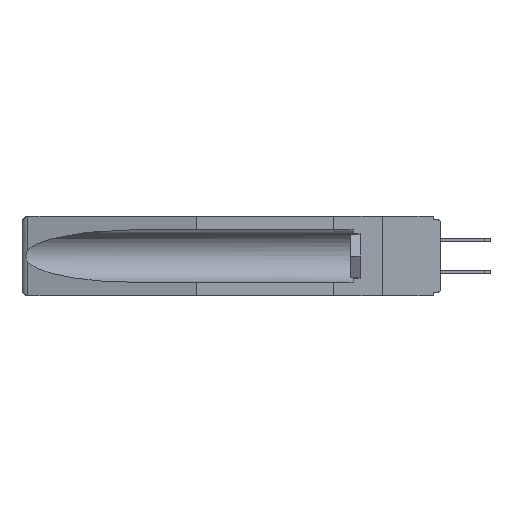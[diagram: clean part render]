
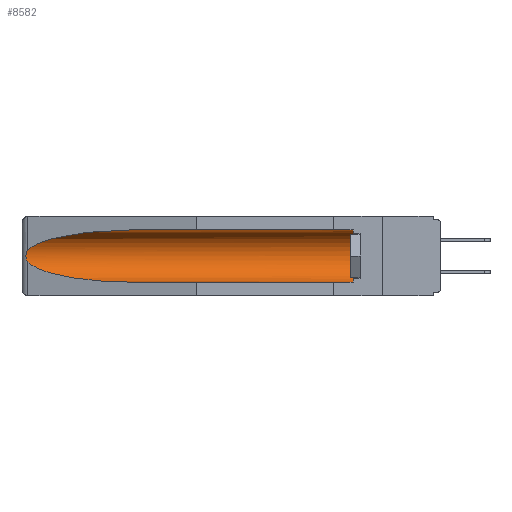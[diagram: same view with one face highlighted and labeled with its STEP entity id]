
A CAD part, left-side view. The second image highlights one B-rep face of the part: STEP entity #8582.
In plain terms, the highlighted cylindrical face has radius 2.857 mm (diameter 5.715 mm), a partial arc.
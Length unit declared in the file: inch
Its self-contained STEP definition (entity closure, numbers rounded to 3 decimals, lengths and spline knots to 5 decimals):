
#1627 = DIRECTION ( 'NONE',  ( 0., -1., 0. ) ) ;
#1773 = CARTESIAN_POINT ( 'NONE',  ( 0.155, -0.30754, -0.1715 ) ) ;
#2093 = AXIS2_PLACEMENT_3D ( 'NONE', #16883, #1627, #15535 ) ;
#2105 = LINE ( 'NONE', #9379, #15382 ) ;
#2114 = CARTESIAN_POINT ( 'NONE',  ( 0.21114, 1.30732, -0.059 ) ) ;
#2133 = CARTESIAN_POINT ( 'NONE',  ( 0.26597, 1.52961, -0.15275 ) ) ;
#2170 = FACE_OUTER_BOUND ( 'NONE', #7596, .T. ) ;
#2476 =( BOUNDED_CURVE ( )  B_SPLINE_CURVE ( 3, ( #14706, #4931, #17585, #3435 ),
 .UNSPECIFIED., .F., .F. ) 
 B_SPLINE_CURVE_WITH_KNOTS ( ( 4, 4 ),
 ( 0.1948, 1.5708 ),
 .UNSPECIFIED. ) 
 CURVE ( )  GEOMETRIC_REPRESENTATION_ITEM ( )  RATIONAL_B_SPLINE_CURVE ( ( 1., 0.848, 0.848, 1. ) ) 
 REPRESENTATION_ITEM ( '' )  );
#2483 = EDGE_CURVE ( 'NONE', #9622, #3540, #13311, .T. ) ;
#2827 = ORIENTED_EDGE ( 'NONE', *, *, #14775, .T. ) ;
#2830 = CYLINDRICAL_SURFACE ( 'NONE', #15640, 0.1125 ) ;
#3435 = CARTESIAN_POINT ( 'NONE',  ( 0.155, 1.07973, -0.284 ) ) ;
#3485 = CARTESIAN_POINT ( 'NONE',  ( 0.26537, 1.52718, -0.19328 ) ) ;
#3540 = VERTEX_POINT ( 'NONE', #5887 ) ;
#3543 = CARTESIAN_POINT ( 'NONE',  ( 0.26654, 1.53092, -0.15636 ) ) ;
#3676 = ORIENTED_EDGE ( 'NONE', *, *, #2483, .T. ) ;
#4139 = DIRECTION ( 'NONE',  ( 0., 1., 0. ) ) ;
#4841 = EDGE_CURVE ( 'NONE', #11686, #8563, #2105, .T. ) ;
#4931 = CARTESIAN_POINT ( 'NONE',  ( 0.25451, 1.48313, -0.24835 ) ) ;
#5887 = CARTESIAN_POINT ( 'NONE',  ( 0.155, 1.07973, -0.059 ) ) ;
#6237 = ORIENTED_EDGE ( 'NONE', *, *, #15553, .T. ) ;
#7541 = CARTESIAN_POINT ( 'NONE',  ( 0.26537, 1.52718, -0.14972 ) ) ;
#7596 = EDGE_LOOP ( 'NONE', ( #9903, #6237, #14422, #8788, #2827, #3676 ) ) ;
#8563 = VERTEX_POINT ( 'NONE', #14243 ) ;
#8582 = ADVANCED_FACE ( 'NONE', ( #2170 ), #2830, .F. ) ;
#8738 = EDGE_CURVE ( 'NONE', #14089, #8563, #2476, .T. ) ;
#8788 = ORIENTED_EDGE ( 'NONE', *, *, #4841, .F. ) ;
#9379 = CARTESIAN_POINT ( 'NONE',  ( 0.155, -0.30754, -0.284 ) ) ;
#9387 = VECTOR ( 'NONE', #4139, 39.37008 ) ;
#9622 = VERTEX_POINT ( 'NONE', #11441 ) ;
#9903 = ORIENTED_EDGE ( 'NONE', *, *, #14136, .T. ) ;
#10482 = B_SPLINE_CURVE_WITH_KNOTS ( 'NONE', 3,
 ( #13209, #2133, #3543, #15940, #17348, #15754, #15999, #11792, #14588, #3485 ),
 .UNSPECIFIED., .F., .F.,
 ( 4, 2, 2, 2, 4 ),
 ( 0., 0.00029, 0.00058, 0.00087, 0.00117 ),
 .UNSPECIFIED. ) ;
#10496 = CARTESIAN_POINT ( 'NONE',  ( 0.155, 1.07973, -0.059 ) ) ;
#10692 = CIRCLE ( 'NONE', #2093, 0.1125 ) ;
#11097 = CARTESIAN_POINT ( 'NONE',  ( 0.155, -0.30754, -0.059 ) ) ;
#11441 = CARTESIAN_POINT ( 'NONE',  ( 0.155, 0.126, -0.059 ) ) ;
#11487 = DIRECTION ( 'NONE',  ( 0., 1., 0. ) ) ;
#11686 = VERTEX_POINT ( 'NONE', #12101 ) ;
#11792 = CARTESIAN_POINT ( 'NONE',  ( 0.26655, 1.53094, -0.18657 ) ) ;
#12101 = CARTESIAN_POINT ( 'NONE',  ( 0.155, 0.126, -0.284 ) ) ;
#12241 = DIRECTION ( 'NONE',  ( 0., 1., 0. ) ) ;
#12649 =( BOUNDED_CURVE ( )  B_SPLINE_CURVE ( 3, ( #10496, #2114, #14518, #16039 ),
 .UNSPECIFIED., .F., .F. ) 
 B_SPLINE_CURVE_WITH_KNOTS ( ( 4, 4 ),
 ( 4.71239, 6.08839 ),
 .UNSPECIFIED. ) 
 CURVE ( )  GEOMETRIC_REPRESENTATION_ITEM ( )  RATIONAL_B_SPLINE_CURVE ( ( 1., 0.848, 0.848, 1. ) ) 
 REPRESENTATION_ITEM ( '' )  );
#13209 = CARTESIAN_POINT ( 'NONE',  ( 0.26537, 1.52718, -0.14972 ) ) ;
#13311 = LINE ( 'NONE', #11097, #9387 ) ;
#14089 = VERTEX_POINT ( 'NONE', #15981 ) ;
#14136 = EDGE_CURVE ( 'NONE', #3540, #15534, #12649, .T. ) ;
#14243 = CARTESIAN_POINT ( 'NONE',  ( 0.155, 1.07973, -0.284 ) ) ;
#14422 = ORIENTED_EDGE ( 'NONE', *, *, #8738, .T. ) ;
#14518 = CARTESIAN_POINT ( 'NONE',  ( 0.25451, 1.48313, -0.09465 ) ) ;
#14588 = CARTESIAN_POINT ( 'NONE',  ( 0.26597, 1.5296, -0.19026 ) ) ;
#14706 = CARTESIAN_POINT ( 'NONE',  ( 0.26537, 1.52718, -0.19328 ) ) ;
#14775 = EDGE_CURVE ( 'NONE', #11686, #9622, #10692, .T. ) ;
#15382 = VECTOR ( 'NONE', #12241, 39.37008 ) ;
#15534 = VERTEX_POINT ( 'NONE', #7541 ) ;
#15535 = DIRECTION ( 'NONE',  ( 0., 0., 1. ) ) ;
#15553 = EDGE_CURVE ( 'NONE', #15534, #14089, #10482, .T. ) ;
#15640 = AXIS2_PLACEMENT_3D ( 'NONE', #1773, #11487, #17095 ) ;
#15754 = CARTESIAN_POINT ( 'NONE',  ( 0.2675, 1.53308, -0.17534 ) ) ;
#15940 = CARTESIAN_POINT ( 'NONE',  ( 0.2673, 1.5327, -0.16383 ) ) ;
#15981 = CARTESIAN_POINT ( 'NONE',  ( 0.26537, 1.52718, -0.19328 ) ) ;
#15999 = CARTESIAN_POINT ( 'NONE',  ( 0.2673, 1.53269, -0.17917 ) ) ;
#16039 = CARTESIAN_POINT ( 'NONE',  ( 0.26537, 1.52718, -0.14972 ) ) ;
#16883 = CARTESIAN_POINT ( 'NONE',  ( 0.155, 0.126, -0.1715 ) ) ;
#17095 = DIRECTION ( 'NONE',  ( 0., 0., 1. ) ) ;
#17348 = CARTESIAN_POINT ( 'NONE',  ( 0.2675, 1.53308, -0.16763 ) ) ;
#17585 = CARTESIAN_POINT ( 'NONE',  ( 0.21114, 1.30732, -0.284 ) ) ;
